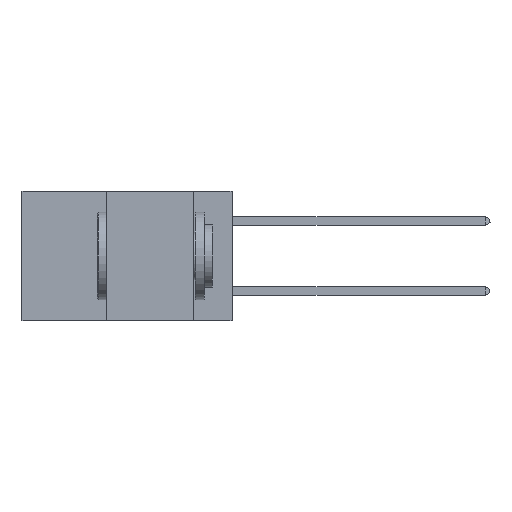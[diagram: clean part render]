
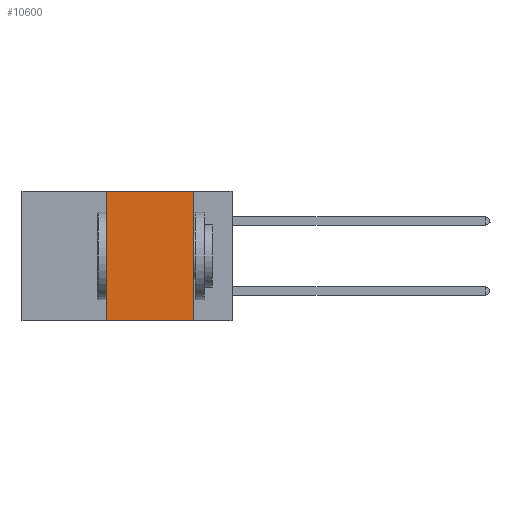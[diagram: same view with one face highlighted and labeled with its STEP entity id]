
A CAD part, left-side view. The second image highlights one B-rep face of the part: STEP entity #10600.
In plain terms, the highlighted planar face has unit normal (-1, 0, 0).
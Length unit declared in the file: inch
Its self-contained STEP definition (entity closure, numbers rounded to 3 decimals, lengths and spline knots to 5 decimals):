
#558 = VECTOR ( 'NONE', #1685, 39.37008 ) ;
#998 = EDGE_CURVE ( 'NONE', #2744, #9491, #9646, .T. ) ;
#1581 = DIRECTION ( 'NONE',  ( 0., 0., -1. ) ) ;
#1685 = DIRECTION ( 'NONE',  ( 0., 0., -1. ) ) ;
#1839 = CARTESIAN_POINT ( 'NONE',  ( 0., 0.11, 0. ) ) ;
#2246 = VERTEX_POINT ( 'NONE', #1839 ) ;
#2677 = CARTESIAN_POINT ( 'NONE',  ( 0., 0.11, -0.37 ) ) ;
#2744 = VERTEX_POINT ( 'NONE', #8490 ) ;
#3397 = LINE ( 'NONE', #3938, #9163 ) ;
#3938 = CARTESIAN_POINT ( 'NONE',  ( 0., 0.6, -0.37 ) ) ;
#4326 = CARTESIAN_POINT ( 'NONE',  ( 0., 0.6, 0. ) ) ;
#5184 = DIRECTION ( 'NONE',  ( 0., -1., 0. ) ) ;
#5647 = ORIENTED_EDGE ( 'NONE', *, *, #998, .F. ) ;
#5724 = CARTESIAN_POINT ( 'NONE',  ( 0., 0.36, 0. ) ) ;
#5820 = VECTOR ( 'NONE', #7080, 39.37008 ) ;
#6011 = PLANE ( 'NONE',  #9249 ) ;
#6051 = FACE_OUTER_BOUND ( 'NONE', #6619, .T. ) ;
#6619 = EDGE_LOOP ( 'NONE', ( #6690, #9964, #5647, #10684 ) ) ;
#6690 = ORIENTED_EDGE ( 'NONE', *, *, #11141, .F. ) ;
#7080 = DIRECTION ( 'NONE',  ( 0., 0., 1. ) ) ;
#7241 = VECTOR ( 'NONE', #10495, 39.37008 ) ;
#7632 = LINE ( 'NONE', #9908, #7241 ) ;
#7788 = VERTEX_POINT ( 'NONE', #2677 ) ;
#8299 = LINE ( 'NONE', #10607, #558 ) ;
#8490 = CARTESIAN_POINT ( 'NONE',  ( 0., 0.36, -0.37 ) ) ;
#8733 = DIRECTION ( 'NONE',  ( 1., 0., 0. ) ) ;
#8839 = EDGE_CURVE ( 'NONE', #9491, #2246, #7632, .T. ) ;
#9163 = VECTOR ( 'NONE', #5184, 39.37008 ) ;
#9249 = AXIS2_PLACEMENT_3D ( 'NONE', #4326, #8733, #1581 ) ;
#9491 = VERTEX_POINT ( 'NONE', #5724 ) ;
#9646 = LINE ( 'NONE', #10579, #5820 ) ;
#9908 = CARTESIAN_POINT ( 'NONE',  ( 0., 0.6, 0. ) ) ;
#9964 = ORIENTED_EDGE ( 'NONE', *, *, #8839, .F. ) ;
#10190 = EDGE_CURVE ( 'NONE', #2744, #7788, #3397, .T. ) ;
#10495 = DIRECTION ( 'NONE',  ( 0., -1., 0. ) ) ;
#10579 = CARTESIAN_POINT ( 'NONE',  ( 0., 0.36, 0. ) ) ;
#10600 = ADVANCED_FACE ( 'NONE', ( #6051 ), #6011, .F. ) ;
#10607 = CARTESIAN_POINT ( 'NONE',  ( 0., 0.11, 0. ) ) ;
#10684 = ORIENTED_EDGE ( 'NONE', *, *, #10190, .T. ) ;
#11141 = EDGE_CURVE ( 'NONE', #2246, #7788, #8299, .T. ) ;
